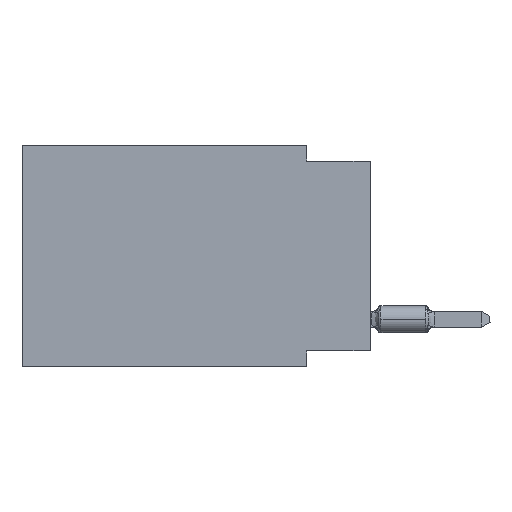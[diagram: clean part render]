
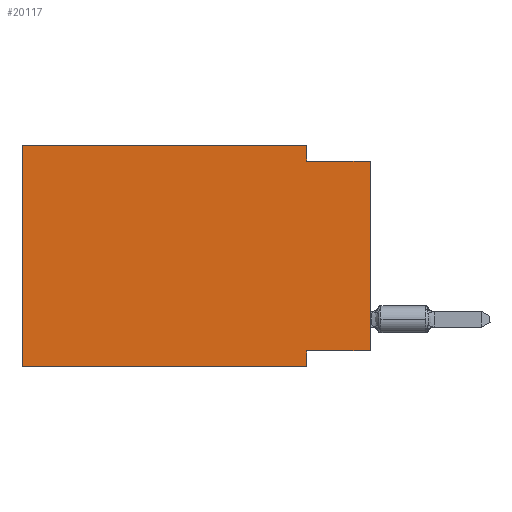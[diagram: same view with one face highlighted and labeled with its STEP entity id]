
A CAD part, left-side view. The second image highlights one B-rep face of the part: STEP entity #20117.
In plain terms, the highlighted planar face has unit normal (-1, 0, 0).
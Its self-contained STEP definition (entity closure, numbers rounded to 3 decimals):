
#909 = VECTOR ( 'NONE', #26231, 1000. ) ;
#1442 = CARTESIAN_POINT ( 'NONE',  ( 0., 2.54, -8.89 ) ) ;
#1744 = DIRECTION ( 'NONE',  ( 0., -1., 0. ) ) ;
#1965 = VERTEX_POINT ( 'NONE', #1442 ) ;
#2031 = CARTESIAN_POINT ( 'NONE',  ( 0., 0., -0.635 ) ) ;
#2055 = DIRECTION ( 'NONE',  ( 0., 0., -1. ) ) ;
#2145 = CARTESIAN_POINT ( 'NONE',  ( 0., 13.97, 0. ) ) ;
#2203 = VERTEX_POINT ( 'NONE', #26840 ) ;
#2331 = ORIENTED_EDGE ( 'NONE', *, *, #5062, .T. ) ;
#2368 = VERTEX_POINT ( 'NONE', #23907 ) ;
#2407 = VERTEX_POINT ( 'NONE', #8280 ) ;
#2411 = CARTESIAN_POINT ( 'NONE',  ( 0., 2.54, 0. ) ) ;
#2812 = LINE ( 'NONE', #4728, #21007 ) ;
#3766 = LINE ( 'NONE', #17352, #15094 ) ;
#3817 = EDGE_CURVE ( 'NONE', #2368, #2407, #25607, .T. ) ;
#3931 = FACE_OUTER_BOUND ( 'NONE', #19735, .T. ) ;
#4236 = LINE ( 'NONE', #2031, #17673 ) ;
#4502 = DIRECTION ( 'NONE',  ( 0., 0., -1. ) ) ;
#4728 = CARTESIAN_POINT ( 'NONE',  ( 0., 13.97, 0. ) ) ;
#5062 = EDGE_CURVE ( 'NONE', #28731, #2203, #3766, .T. ) ;
#6136 = ORIENTED_EDGE ( 'NONE', *, *, #8988, .T. ) ;
#8154 = DIRECTION ( 'NONE',  ( 0., 0., 1. ) ) ;
#8161 = CARTESIAN_POINT ( 'NONE',  ( 0., 2.54, -0.635 ) ) ;
#8280 = CARTESIAN_POINT ( 'NONE',  ( 0., 2.54, 0. ) ) ;
#8336 = VERTEX_POINT ( 'NONE', #8161 ) ;
#8398 = LINE ( 'NONE', #15252, #21408 ) ;
#8988 = EDGE_CURVE ( 'NONE', #13982, #1965, #8398, .T. ) ;
#9125 = CARTESIAN_POINT ( 'NONE',  ( 0., 2.54, -8.255 ) ) ;
#9698 = DIRECTION ( 'NONE',  ( 0., -1., 0. ) ) ;
#9758 = VECTOR ( 'NONE', #9698, 1000. ) ;
#9793 = EDGE_CURVE ( 'NONE', #8336, #2203, #4236, .T. ) ;
#10085 = VERTEX_POINT ( 'NONE', #9125 ) ;
#10722 = VECTOR ( 'NONE', #2055, 1000. ) ;
#11050 = EDGE_CURVE ( 'NONE', #10085, #1965, #13020, .T. ) ;
#11847 = CARTESIAN_POINT ( 'NONE',  ( 0., 0., -8.255 ) ) ;
#11901 = CARTESIAN_POINT ( 'NONE',  ( 0., 13.97, 0. ) ) ;
#13020 = LINE ( 'NONE', #15351, #10722 ) ;
#13077 = ORIENTED_EDGE ( 'NONE', *, *, #11050, .F. ) ;
#13316 = VECTOR ( 'NONE', #22918, 1000. ) ;
#13982 = VERTEX_POINT ( 'NONE', #28216 ) ;
#14206 = ORIENTED_EDGE ( 'NONE', *, *, #15568, .F. ) ;
#14311 = LINE ( 'NONE', #27300, #13316 ) ;
#15094 = VECTOR ( 'NONE', #8154, 1000. ) ;
#15252 = CARTESIAN_POINT ( 'NONE',  ( 0., 13.97, -8.89 ) ) ;
#15351 = CARTESIAN_POINT ( 'NONE',  ( 0., 2.54, -8.89 ) ) ;
#15568 = EDGE_CURVE ( 'NONE', #28731, #10085, #14311, .T. ) ;
#16104 = DIRECTION ( 'NONE',  ( 0., 0., 1. ) ) ;
#17244 = ORIENTED_EDGE ( 'NONE', *, *, #18107, .F. ) ;
#17311 = DIRECTION ( 'NONE',  ( 0., -1., 0. ) ) ;
#17352 = CARTESIAN_POINT ( 'NONE',  ( 0., 0., 0. ) ) ;
#17531 = EDGE_CURVE ( 'NONE', #2407, #8336, #26368, .T. ) ;
#17673 = VECTOR ( 'NONE', #1744, 1000. ) ;
#18107 = EDGE_CURVE ( 'NONE', #13982, #2368, #2812, .T. ) ;
#18435 = ORIENTED_EDGE ( 'NONE', *, *, #17531, .F. ) ;
#19735 = EDGE_LOOP ( 'NONE', ( #2331, #23369, #18435, #24142, #17244, #6136, #13077, #14206 ) ) ;
#20117 = ADVANCED_FACE ( 'NONE', ( #3931 ), #21878, .F. ) ;
#20580 = AXIS2_PLACEMENT_3D ( 'NONE', #2145, #28303, #4502 ) ;
#21007 = VECTOR ( 'NONE', #16104, 1000. ) ;
#21408 = VECTOR ( 'NONE', #17311, 1000. ) ;
#21878 = PLANE ( 'NONE',  #20580 ) ;
#22918 = DIRECTION ( 'NONE',  ( 0., 1., 0. ) ) ;
#23369 = ORIENTED_EDGE ( 'NONE', *, *, #9793, .F. ) ;
#23907 = CARTESIAN_POINT ( 'NONE',  ( 0., 13.97, 0. ) ) ;
#24142 = ORIENTED_EDGE ( 'NONE', *, *, #3817, .F. ) ;
#25607 = LINE ( 'NONE', #11901, #9758 ) ;
#26231 = DIRECTION ( 'NONE',  ( 0., 0., -1. ) ) ;
#26368 = LINE ( 'NONE', #2411, #909 ) ;
#26840 = CARTESIAN_POINT ( 'NONE',  ( 0., 0., -0.635 ) ) ;
#27300 = CARTESIAN_POINT ( 'NONE',  ( 0., 0., -8.255 ) ) ;
#28216 = CARTESIAN_POINT ( 'NONE',  ( 0., 13.97, -8.89 ) ) ;
#28303 = DIRECTION ( 'NONE',  ( 1., 0., 0. ) ) ;
#28731 = VERTEX_POINT ( 'NONE', #11847 ) ;
